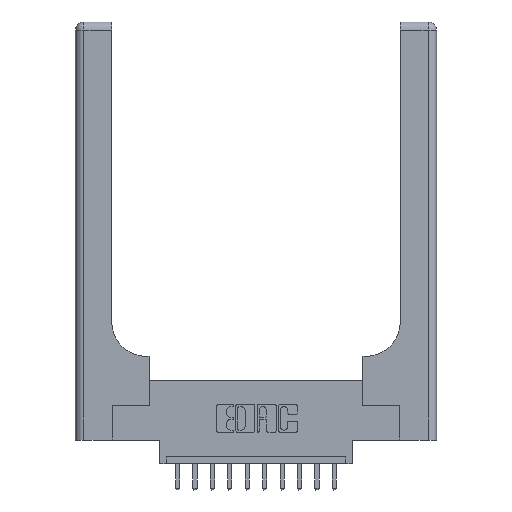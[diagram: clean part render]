
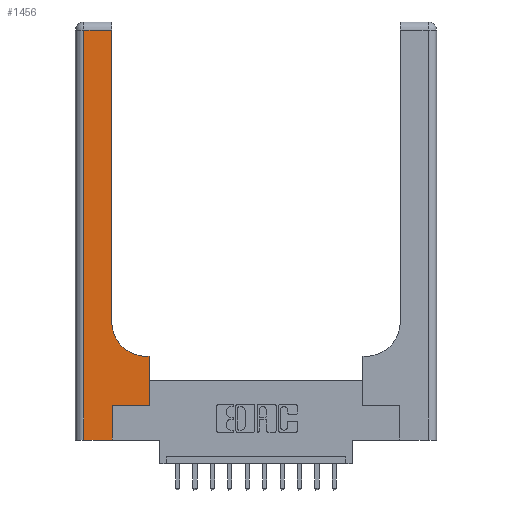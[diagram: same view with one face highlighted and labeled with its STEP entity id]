
A CAD part, top view. The second image highlights one B-rep face of the part: STEP entity #1456.
In plain terms, the highlighted planar face has unit normal (0, 0, 1).
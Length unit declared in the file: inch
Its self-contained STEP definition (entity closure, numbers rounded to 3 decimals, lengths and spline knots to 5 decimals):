
#86 = AXIS2_PLACEMENT_3D ( 'NONE', #2681, #9859, #12461 ) ;
#415 = ORIENTED_EDGE ( 'NONE', *, *, #843, .T. ) ;
#657 = ORIENTED_EDGE ( 'NONE', *, *, #14517, .T. ) ;
#712 = VERTEX_POINT ( 'NONE', #10773 ) ;
#747 = VECTOR ( 'NONE', #13558, 39.37008 ) ;
#843 = EDGE_CURVE ( 'NONE', #14896, #712, #8951, .T. ) ;
#855 = LINE ( 'NONE', #11700, #2792 ) ;
#1456 = ADVANCED_FACE ( 'NONE', ( #12597 ), #5393, .F. ) ;
#1500 = CARTESIAN_POINT ( 'NONE',  ( 0.06, 2.94, 0.37 ) ) ;
#1861 = DIRECTION ( 'NONE',  ( -1., 0., 0. ) ) ;
#2364 = CARTESIAN_POINT ( 'NONE',  ( 0., 2.94, 0.37 ) ) ;
#2520 = CARTESIAN_POINT ( 'NONE',  ( 0.265, 0.25, 0.37 ) ) ;
#2681 = CARTESIAN_POINT ( 'NONE',  ( 0.51, 0.85, 0.37 ) ) ;
#2792 = VECTOR ( 'NONE', #7813, 39.37008 ) ;
#2822 = LINE ( 'NONE', #13450, #12686 ) ;
#2837 = CARTESIAN_POINT ( 'NONE',  ( 0.528, 0.25, 0.37 ) ) ;
#3611 = DIRECTION ( 'NONE',  ( 0., -1., 0. ) ) ;
#3738 = LINE ( 'NONE', #2364, #8204 ) ;
#3848 = CARTESIAN_POINT ( 'NONE',  ( 0.51, 0.6, 0.37 ) ) ;
#4306 = EDGE_CURVE ( 'NONE', #5450, #7688, #12509, .T. ) ;
#4505 = ORIENTED_EDGE ( 'NONE', *, *, #4306, .T. ) ;
#4797 = CARTESIAN_POINT ( 'NONE',  ( 0.06, 0., 0.37 ) ) ;
#4870 = EDGE_CURVE ( 'NONE', #14925, #9034, #2822, .T. ) ;
#4889 = CARTESIAN_POINT ( 'NONE',  ( 0.265, 0.25, 0.37 ) ) ;
#5033 = CARTESIAN_POINT ( 'NONE',  ( 0.528, 0.25, 0.37 ) ) ;
#5119 = ORIENTED_EDGE ( 'NONE', *, *, #11742, .T. ) ;
#5165 = VERTEX_POINT ( 'NONE', #2520 ) ;
#5205 = CARTESIAN_POINT ( 'NONE',  ( 0., 0., 0.37 ) ) ;
#5393 = PLANE ( 'NONE',  #8743 ) ;
#5399 = CARTESIAN_POINT ( 'NONE',  ( 0.26, 3., 0.37 ) ) ;
#5450 = VERTEX_POINT ( 'NONE', #3848 ) ;
#5502 = CARTESIAN_POINT ( 'NONE',  ( 0., 3., 0.37 ) ) ;
#5733 = DIRECTION ( 'NONE',  ( 0., 1., 0. ) ) ;
#5831 = VECTOR ( 'NONE', #9845, 39.37008 ) ;
#5905 = CARTESIAN_POINT ( 'NONE',  ( 0.265, 0., 0.37 ) ) ;
#5955 = EDGE_CURVE ( 'NONE', #9034, #8273, #14388, .T. ) ;
#6481 = VECTOR ( 'NONE', #13898, 39.37008 ) ;
#6635 = ORIENTED_EDGE ( 'NONE', *, *, #9686, .T. ) ;
#6799 = VECTOR ( 'NONE', #5733, 39.37008 ) ;
#7688 = VERTEX_POINT ( 'NONE', #9670 ) ;
#7813 = DIRECTION ( 'NONE',  ( -1., 0., 0. ) ) ;
#7952 = ORIENTED_EDGE ( 'NONE', *, *, #4870, .T. ) ;
#8204 = VECTOR ( 'NONE', #9696, 39.37008 ) ;
#8256 = CARTESIAN_POINT ( 'NONE',  ( 0.265, 0., 0.37 ) ) ;
#8273 = VERTEX_POINT ( 'NONE', #8256 ) ;
#8362 = LINE ( 'NONE', #5399, #6799 ) ;
#8743 = AXIS2_PLACEMENT_3D ( 'NONE', #5502, #14135, #1861 ) ;
#8951 = LINE ( 'NONE', #5033, #5831 ) ;
#9034 = VERTEX_POINT ( 'NONE', #4797 ) ;
#9358 = ORIENTED_EDGE ( 'NONE', *, *, #14739, .T. ) ;
#9670 = CARTESIAN_POINT ( 'NONE',  ( 0.26, 0.85, 0.37 ) ) ;
#9686 = EDGE_CURVE ( 'NONE', #5165, #14896, #14946, .T. ) ;
#9696 = DIRECTION ( 'NONE',  ( -1., 0., 0. ) ) ;
#9845 = DIRECTION ( 'NONE',  ( 0., 1., 0. ) ) ;
#9859 = DIRECTION ( 'NONE',  ( 0., 0., -1. ) ) ;
#9975 = DIRECTION ( 'NONE',  ( 1., 0., 0. ) ) ;
#10452 = VERTEX_POINT ( 'NONE', #12989 ) ;
#10773 = CARTESIAN_POINT ( 'NONE',  ( 0.528, 0.6, 0.37 ) ) ;
#11092 = ORIENTED_EDGE ( 'NONE', *, *, #13150, .T. ) ;
#11700 = CARTESIAN_POINT ( 'NONE',  ( 0.26, 0.6, 0.37 ) ) ;
#11742 = EDGE_CURVE ( 'NONE', #7688, #10452, #8362, .T. ) ;
#12345 = LINE ( 'NONE', #5905, #747 ) ;
#12461 = DIRECTION ( 'NONE',  ( 1., 0., 0. ) ) ;
#12509 = CIRCLE ( 'NONE', #86, 0.25 ) ;
#12597 = FACE_OUTER_BOUND ( 'NONE', #12883, .T. ) ;
#12686 = VECTOR ( 'NONE', #3611, 39.37008 ) ;
#12703 = ORIENTED_EDGE ( 'NONE', *, *, #5955, .T. ) ;
#12883 = EDGE_LOOP ( 'NONE', ( #5119, #9358, #7952, #12703, #11092, #6635, #415, #657, #4505 ) ) ;
#12989 = CARTESIAN_POINT ( 'NONE',  ( 0.26, 2.94, 0.37 ) ) ;
#13150 = EDGE_CURVE ( 'NONE', #8273, #5165, #12345, .T. ) ;
#13450 = CARTESIAN_POINT ( 'NONE',  ( 0.06, 3., 0.37 ) ) ;
#13558 = DIRECTION ( 'NONE',  ( 0., 1., 0. ) ) ;
#13898 = DIRECTION ( 'NONE',  ( 1., 0., 0. ) ) ;
#14000 = VECTOR ( 'NONE', #9975, 39.37008 ) ;
#14135 = DIRECTION ( 'NONE',  ( 0., 0., -1. ) ) ;
#14388 = LINE ( 'NONE', #5205, #6481 ) ;
#14517 = EDGE_CURVE ( 'NONE', #712, #5450, #855, .T. ) ;
#14739 = EDGE_CURVE ( 'NONE', #10452, #14925, #3738, .T. ) ;
#14896 = VERTEX_POINT ( 'NONE', #2837 ) ;
#14925 = VERTEX_POINT ( 'NONE', #1500 ) ;
#14946 = LINE ( 'NONE', #4889, #14000 ) ;
